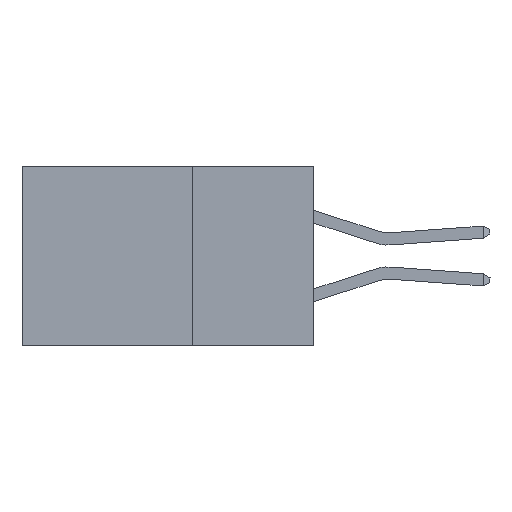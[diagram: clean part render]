
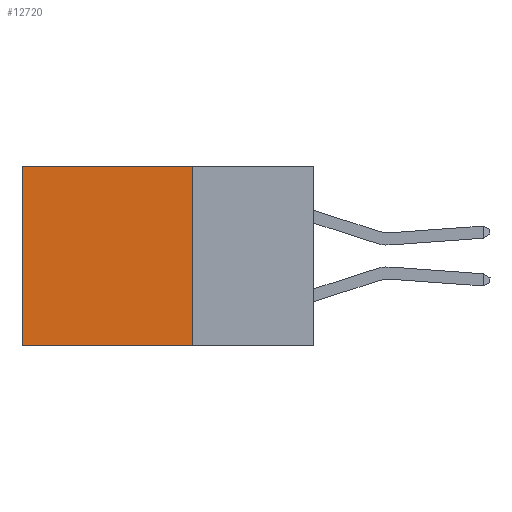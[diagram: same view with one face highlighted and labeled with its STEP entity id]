
A CAD part, left-side view. The second image highlights one B-rep face of the part: STEP entity #12720.
In plain terms, the highlighted planar face has unit normal (-1, 0, 0).
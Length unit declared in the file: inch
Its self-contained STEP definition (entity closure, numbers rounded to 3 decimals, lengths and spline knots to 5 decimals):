
#42 = CARTESIAN_POINT ( 'NONE',  ( 0.2875, 0.25, 0. ) ) ;
#571 = VERTEX_POINT ( 'NONE', #42 ) ;
#1131 = DIRECTION ( 'NONE',  ( 1., 0., 0. ) ) ;
#1734 = VECTOR ( 'NONE', #36242, 39.37008 ) ;
#3785 = ORIENTED_EDGE ( 'NONE', *, *, #36629, .T. ) ;
#4536 = ORIENTED_EDGE ( 'NONE', *, *, #15097, .F. ) ;
#8965 = CARTESIAN_POINT ( 'NONE',  ( 0.2875, 0.25, 0. ) ) ;
#9830 = DIRECTION ( 'NONE',  ( 0., 0., -1. ) ) ;
#10166 = EDGE_CURVE ( 'NONE', #571, #32678, #20525, .T. ) ;
#10538 = VERTEX_POINT ( 'NONE', #30232 ) ;
#12251 = CARTESIAN_POINT ( 'NONE',  ( 0.2875, 0.25, 0. ) ) ;
#12483 = CARTESIAN_POINT ( 'NONE',  ( 0.2875, 0.25, 0. ) ) ;
#12690 = AXIS2_PLACEMENT_3D ( 'NONE', #12251, #1131, #9830 ) ;
#12720 = ADVANCED_FACE ( 'NONE', ( #22307 ), #29604, .F. ) ;
#12900 = ORIENTED_EDGE ( 'NONE', *, *, #34093, .F. ) ;
#13049 = VECTOR ( 'NONE', #18814, 39.37008 ) ;
#13950 = LINE ( 'NONE', #12483, #13049 ) ;
#15097 = EDGE_CURVE ( 'NONE', #571, #26786, #13950, .T. ) ;
#16321 = LINE ( 'NONE', #33093, #1734 ) ;
#16376 = CARTESIAN_POINT ( 'NONE',  ( 0.2875, 0.6, 0. ) ) ;
#16930 = ORIENTED_EDGE ( 'NONE', *, *, #10166, .T. ) ;
#17580 = CARTESIAN_POINT ( 'NONE',  ( 0.2875, 0.25, -0.37 ) ) ;
#18814 = DIRECTION ( 'NONE',  ( 0., 0., -1. ) ) ;
#20525 = LINE ( 'NONE', #8965, #31386 ) ;
#22307 = FACE_OUTER_BOUND ( 'NONE', #30826, .T. ) ;
#26150 = LINE ( 'NONE', #16376, #36571 ) ;
#26468 = DIRECTION ( 'NONE',  ( 0., 1., 0. ) ) ;
#26786 = VERTEX_POINT ( 'NONE', #17580 ) ;
#29604 = PLANE ( 'NONE',  #12690 ) ;
#30232 = CARTESIAN_POINT ( 'NONE',  ( 0.2875, 0.6, -0.37 ) ) ;
#30826 = EDGE_LOOP ( 'NONE', ( #3785, #12900, #4536, #16930 ) ) ;
#31182 = CARTESIAN_POINT ( 'NONE',  ( 0.2875, 0.6, 0. ) ) ;
#31386 = VECTOR ( 'NONE', #26468, 39.37008 ) ;
#32678 = VERTEX_POINT ( 'NONE', #31182 ) ;
#33093 = CARTESIAN_POINT ( 'NONE',  ( 0.2875, 0.25, -0.37 ) ) ;
#34093 = EDGE_CURVE ( 'NONE', #26786, #10538, #16321, .T. ) ;
#36109 = DIRECTION ( 'NONE',  ( 0., 0., -1. ) ) ;
#36242 = DIRECTION ( 'NONE',  ( 0., 1., 0. ) ) ;
#36571 = VECTOR ( 'NONE', #36109, 39.37008 ) ;
#36629 = EDGE_CURVE ( 'NONE', #32678, #10538, #26150, .T. ) ;
